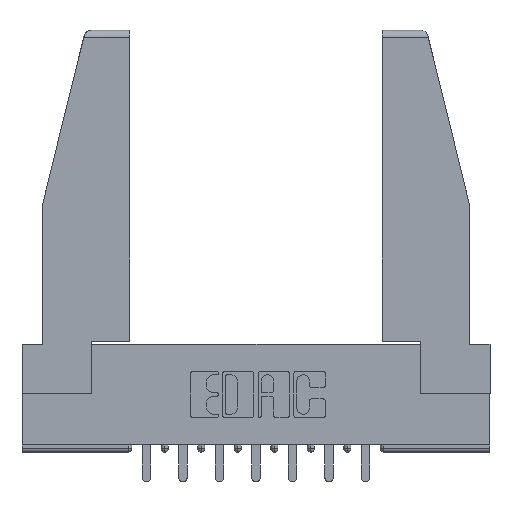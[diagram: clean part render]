
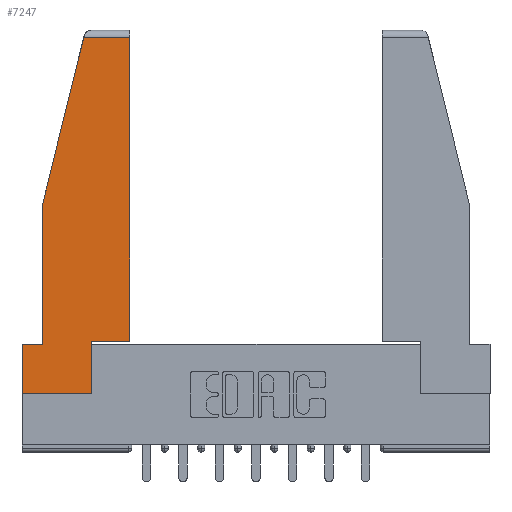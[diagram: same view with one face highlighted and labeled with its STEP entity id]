
A CAD part, top view. The second image highlights one B-rep face of the part: STEP entity #7247.
In plain terms, the highlighted planar face has unit normal (0, 0, 1).
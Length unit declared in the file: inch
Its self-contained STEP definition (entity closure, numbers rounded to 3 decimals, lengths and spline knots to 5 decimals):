
#11 = DIRECTION ( 'NONE',  ( -1., 0., 0. ) ) ;
#75 = EDGE_CURVE ( 'NONE', #121, #8089, #6644, .T. ) ;
#121 = VERTEX_POINT ( 'NONE', #1381 ) ;
#131 = VERTEX_POINT ( 'NONE', #1444 ) ;
#282 = CARTESIAN_POINT ( 'NONE',  ( 0., 1.52, 0. ) ) ;
#317 = ORIENTED_EDGE ( 'NONE', *, *, #2217, .T. ) ;
#808 = LINE ( 'NONE', #3128, #4741 ) ;
#979 = ORIENTED_EDGE ( 'NONE', *, *, #1128, .T. ) ;
#1128 = EDGE_CURVE ( 'NONE', #12443, #8229, #4389, .T. ) ;
#1168 = VECTOR ( 'NONE', #2374, 39.37008 ) ;
#1183 = VECTOR ( 'NONE', #11682, 39.37008 ) ;
#1381 = CARTESIAN_POINT ( 'NONE',  ( 0.297, 0., 0. ) ) ;
#1444 = CARTESIAN_POINT ( 'NONE',  ( 0.2636, 1.52, 0. ) ) ;
#2102 = LINE ( 'NONE', #12273, #7568 ) ;
#2133 = VECTOR ( 'NONE', #11677, 39.37008 ) ;
#2217 = EDGE_CURVE ( 'NONE', #131, #7384, #10942, .T. ) ;
#2374 = DIRECTION ( 'NONE',  ( 1., 0., 0. ) ) ;
#2581 = ORIENTED_EDGE ( 'NONE', *, *, #2674, .T. ) ;
#2600 = DIRECTION ( 'NONE',  ( 0., 1., 0. ) ) ;
#2610 = EDGE_CURVE ( 'NONE', #8229, #121, #808, .T. ) ;
#2626 = VERTEX_POINT ( 'NONE', #5110 ) ;
#2674 = EDGE_CURVE ( 'NONE', #2626, #131, #5456, .T. ) ;
#2777 = VECTOR ( 'NONE', #11776, 39.37008 ) ;
#2828 = ORIENTED_EDGE ( 'NONE', *, *, #3360, .T. ) ;
#2947 = ORIENTED_EDGE ( 'NONE', *, *, #75, .T. ) ;
#3104 = EDGE_CURVE ( 'NONE', #8089, #10480, #11799, .T. ) ;
#3128 = CARTESIAN_POINT ( 'NONE',  ( 0., 0., 0. ) ) ;
#3179 = VECTOR ( 'NONE', #2600, 39.37008 ) ;
#3239 = DIRECTION ( 'NONE',  ( 0., -1., 0. ) ) ;
#3346 = AXIS2_PLACEMENT_3D ( 'NONE', #11143, #10253, #9980 ) ;
#3360 = EDGE_CURVE ( 'NONE', #7384, #11020, #12719, .T. ) ;
#3662 = CARTESIAN_POINT ( 'NONE',  ( 0., 0.21, 0. ) ) ;
#3735 = CARTESIAN_POINT ( 'NONE',  ( 0., 0., 0. ) ) ;
#4389 = LINE ( 'NONE', #12583, #8701 ) ;
#4741 = VECTOR ( 'NONE', #7299, 39.37008 ) ;
#4796 = PLANE ( 'NONE',  #3346 ) ;
#5110 = CARTESIAN_POINT ( 'NONE',  ( 0.461, 1.52, 0. ) ) ;
#5456 = LINE ( 'NONE', #282, #2133 ) ;
#5466 = ORIENTED_EDGE ( 'NONE', *, *, #10847, .T. ) ;
#5518 = CARTESIAN_POINT ( 'NONE',  ( 0.461, 0.223, 0. ) ) ;
#6435 = CARTESIAN_POINT ( 'NONE',  ( 0.086, 0.8, 0. ) ) ;
#6476 = ORIENTED_EDGE ( 'NONE', *, *, #3104, .T. ) ;
#6644 = LINE ( 'NONE', #12853, #3179 ) ;
#6989 = FACE_OUTER_BOUND ( 'NONE', #10374, .T. ) ;
#7247 = ADVANCED_FACE ( 'NONE', ( #6989 ), #4796, .T. ) ;
#7299 = DIRECTION ( 'NONE',  ( 1., 0., 0. ) ) ;
#7384 = VERTEX_POINT ( 'NONE', #6435 ) ;
#7559 = EDGE_CURVE ( 'NONE', #10480, #2626, #10724, .T. ) ;
#7563 = CARTESIAN_POINT ( 'NONE',  ( 0.297, 0.223, 0. ) ) ;
#7568 = VECTOR ( 'NONE', #11, 39.37008 ) ;
#7632 = ORIENTED_EDGE ( 'NONE', *, *, #7559, .T. ) ;
#8089 = VERTEX_POINT ( 'NONE', #9613 ) ;
#8229 = VERTEX_POINT ( 'NONE', #3735 ) ;
#8352 = DIRECTION ( 'NONE',  ( 0., -1., 0. ) ) ;
#8701 = VECTOR ( 'NONE', #3239, 39.37008 ) ;
#9613 = CARTESIAN_POINT ( 'NONE',  ( 0.297, 0.223, 0. ) ) ;
#9708 = CARTESIAN_POINT ( 'NONE',  ( 0.271, 1.55, 0. ) ) ;
#9826 = CARTESIAN_POINT ( 'NONE',  ( 0.461, 0.223, 0. ) ) ;
#9980 = DIRECTION ( 'NONE',  ( 1., 0., 0. ) ) ;
#10253 = DIRECTION ( 'NONE',  ( 0., 0., 1. ) ) ;
#10286 = VECTOR ( 'NONE', #8352, 39.37008 ) ;
#10374 = EDGE_LOOP ( 'NONE', ( #7632, #2581, #317, #2828, #5466, #979, #11470, #2947, #6476 ) ) ;
#10405 = CARTESIAN_POINT ( 'NONE',  ( 0.086, 0.8, 0. ) ) ;
#10480 = VERTEX_POINT ( 'NONE', #5518 ) ;
#10724 = LINE ( 'NONE', #9826, #1183 ) ;
#10847 = EDGE_CURVE ( 'NONE', #11020, #12443, #2102, .T. ) ;
#10942 = LINE ( 'NONE', #9708, #2777 ) ;
#11020 = VERTEX_POINT ( 'NONE', #12045 ) ;
#11143 = CARTESIAN_POINT ( 'NONE',  ( 0., 0., 0. ) ) ;
#11470 = ORIENTED_EDGE ( 'NONE', *, *, #2610, .T. ) ;
#11677 = DIRECTION ( 'NONE',  ( -1., 0., 0. ) ) ;
#11682 = DIRECTION ( 'NONE',  ( 0., 1., 0. ) ) ;
#11776 = DIRECTION ( 'NONE',  ( -0.239, -0.971, 0. ) ) ;
#11799 = LINE ( 'NONE', #7563, #1168 ) ;
#12045 = CARTESIAN_POINT ( 'NONE',  ( 0.086, 0.21, 0. ) ) ;
#12273 = CARTESIAN_POINT ( 'NONE',  ( 0., 0.21, 0. ) ) ;
#12443 = VERTEX_POINT ( 'NONE', #3662 ) ;
#12583 = CARTESIAN_POINT ( 'NONE',  ( 0., 0.21, 0. ) ) ;
#12719 = LINE ( 'NONE', #10405, #10286 ) ;
#12853 = CARTESIAN_POINT ( 'NONE',  ( 0.297, 0., 0. ) ) ;
